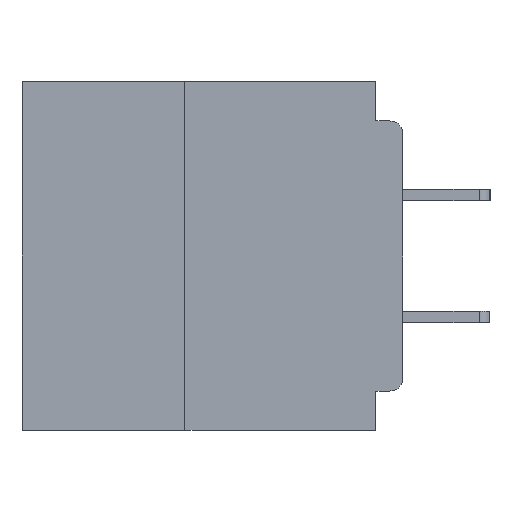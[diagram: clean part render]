
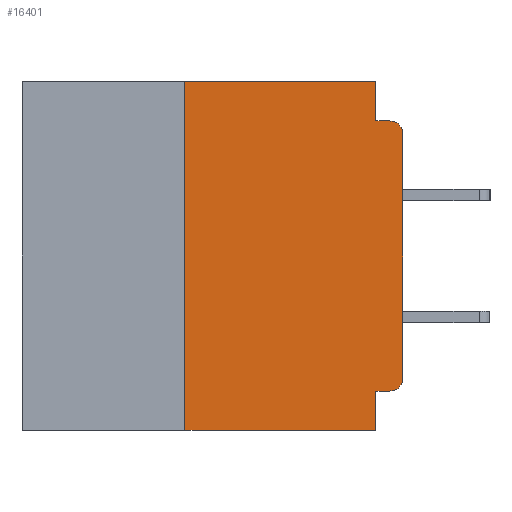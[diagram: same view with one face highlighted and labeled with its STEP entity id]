
A CAD part, left-side view. The second image highlights one B-rep face of the part: STEP entity #16401.
In plain terms, the highlighted planar face has unit normal (-1, 0, 0).
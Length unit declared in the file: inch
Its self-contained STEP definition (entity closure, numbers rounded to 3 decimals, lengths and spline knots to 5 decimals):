
#116 = ORIENTED_EDGE ( 'NONE', *, *, #17835, .T. ) ;
#243 = DIRECTION ( 'NONE',  ( 1., 0., 0. ) ) ;
#404 = ORIENTED_EDGE ( 'NONE', *, *, #12622, .F. ) ;
#516 = DIRECTION ( 'NONE',  ( 0., -1., 0. ) ) ;
#699 = ORIENTED_EDGE ( 'NONE', *, *, #6581, .F. ) ;
#731 = CARTESIAN_POINT ( 'NONE',  ( 0., 0.437, 0. ) ) ;
#815 = CARTESIAN_POINT ( 'NONE',  ( 0., 0.031, -0.355 ) ) ;
#990 = VECTOR ( 'NONE', #34833, 39.37008 ) ;
#2074 = EDGE_CURVE ( 'NONE', #23685, #32540, #9881, .T. ) ;
#2911 = EDGE_CURVE ( 'NONE', #17090, #6119, #20138, .T. ) ;
#3537 = CARTESIAN_POINT ( 'NONE',  ( 0., 0.031, 0. ) ) ;
#3627 = EDGE_CURVE ( 'NONE', #30890, #26163, #35342, .T. ) ;
#3817 = FACE_OUTER_BOUND ( 'NONE', #31645, .T. ) ;
#4033 = CARTESIAN_POINT ( 'NONE',  ( 0., 0.015, -0.355 ) ) ;
#4308 = ORIENTED_EDGE ( 'NONE', *, *, #5670, .F. ) ;
#4828 = ORIENTED_EDGE ( 'NONE', *, *, #32308, .F. ) ;
#4976 = VERTEX_POINT ( 'NONE', #22379 ) ;
#5037 = VECTOR ( 'NONE', #11002, 39.37008 ) ;
#5136 = VECTOR ( 'NONE', #11388, 39.37008 ) ;
#5670 = EDGE_CURVE ( 'NONE', #26163, #34855, #36086, .T. ) ;
#6070 = CARTESIAN_POINT ( 'NONE',  ( 0., 0.437, 0. ) ) ;
#6119 = VERTEX_POINT ( 'NONE', #20509 ) ;
#6156 = DIRECTION ( 'NONE',  ( -1., 0., 0. ) ) ;
#6455 = CARTESIAN_POINT ( 'NONE',  ( 0., 0.437, -0.4 ) ) ;
#6581 = EDGE_CURVE ( 'NONE', #4976, #35070, #22081, .T. ) ;
#9729 = CARTESIAN_POINT ( 'NONE',  ( 0., 0.031, -0.4 ) ) ;
#9881 = LINE ( 'NONE', #731, #30700 ) ;
#9949 = AXIS2_PLACEMENT_3D ( 'NONE', #23336, #6156, #26182 ) ;
#11002 = DIRECTION ( 'NONE',  ( 0., 0., -1. ) ) ;
#11388 = DIRECTION ( 'NONE',  ( 0., 1., 0. ) ) ;
#11932 = CARTESIAN_POINT ( 'NONE',  ( 0., 0., -0.355 ) ) ;
#12227 = ORIENTED_EDGE ( 'NONE', *, *, #3627, .F. ) ;
#12308 = LINE ( 'NONE', #6455, #25605 ) ;
#12622 = EDGE_CURVE ( 'NONE', #32540, #4976, #33221, .T. ) ;
#13429 = CARTESIAN_POINT ( 'NONE',  ( 0., 0.25, -0.4 ) ) ;
#13661 = VECTOR ( 'NONE', #23014, 39.37008 ) ;
#15218 = DIRECTION ( 'NONE',  ( 0., 0., 1. ) ) ;
#15325 = CARTESIAN_POINT ( 'NONE',  ( 0., 0.25, 0. ) ) ;
#15839 = DIRECTION ( 'NONE',  ( -1., 0., 0. ) ) ;
#16401 = ADVANCED_FACE ( 'NONE', ( #3817 ), #28958, .F. ) ;
#16476 = ORIENTED_EDGE ( 'NONE', *, *, #19208, .T. ) ;
#17090 = VERTEX_POINT ( 'NONE', #26309 ) ;
#17835 = EDGE_CURVE ( 'NONE', #6119, #35070, #34373, .T. ) ;
#18929 = ORIENTED_EDGE ( 'NONE', *, *, #35498, .T. ) ;
#19208 = EDGE_CURVE ( 'NONE', #28558, #34855, #12308, .T. ) ;
#19770 = VECTOR ( 'NONE', #15218, 39.37008 ) ;
#20138 = LINE ( 'NONE', #24200, #26715 ) ;
#20509 = CARTESIAN_POINT ( 'NONE',  ( 0., 0., -0.06 ) ) ;
#20597 = DIRECTION ( 'NONE',  ( 0., 0., -1. ) ) ;
#20950 = DIRECTION ( 'NONE',  ( 0., -1., 0. ) ) ;
#21707 = ORIENTED_EDGE ( 'NONE', *, *, #2911, .T. ) ;
#22081 = LINE ( 'NONE', #36866, #13661 ) ;
#22379 = CARTESIAN_POINT ( 'NONE',  ( 0., 0.031, -0.045 ) ) ;
#23014 = DIRECTION ( 'NONE',  ( 0., -1., 0. ) ) ;
#23336 = CARTESIAN_POINT ( 'NONE',  ( 0., 0.015, -0.06 ) ) ;
#23685 = VERTEX_POINT ( 'NONE', #15325 ) ;
#23905 = DIRECTION ( 'NONE',  ( 0., 0., 1. ) ) ;
#24200 = CARTESIAN_POINT ( 'NONE',  ( 0., 0., 0. ) ) ;
#24721 = CIRCLE ( 'NONE', #29258, 0.015 ) ;
#24935 = CARTESIAN_POINT ( 'NONE',  ( 0., 0.031, 0. ) ) ;
#25605 = VECTOR ( 'NONE', #20950, 39.37008 ) ;
#26163 = VERTEX_POINT ( 'NONE', #815 ) ;
#26182 = DIRECTION ( 'NONE',  ( 0., 0., -1. ) ) ;
#26309 = CARTESIAN_POINT ( 'NONE',  ( 0., 0., -0.34 ) ) ;
#26715 = VECTOR ( 'NONE', #23905, 39.37008 ) ;
#26828 = AXIS2_PLACEMENT_3D ( 'NONE', #6070, #243, #20597 ) ;
#27618 = LINE ( 'NONE', #34825, #19770 ) ;
#28558 = VERTEX_POINT ( 'NONE', #13429 ) ;
#28958 = PLANE ( 'NONE',  #26828 ) ;
#29258 = AXIS2_PLACEMENT_3D ( 'NONE', #32672, #15839, #35416 ) ;
#29561 = ORIENTED_EDGE ( 'NONE', *, *, #2074, .F. ) ;
#30700 = VECTOR ( 'NONE', #516, 39.37008 ) ;
#30890 = VERTEX_POINT ( 'NONE', #4033 ) ;
#31645 = EDGE_LOOP ( 'NONE', ( #21707, #116, #699, #404, #29561, #4828, #16476, #4308, #12227, #18929 ) ) ;
#32308 = EDGE_CURVE ( 'NONE', #28558, #23685, #27618, .T. ) ;
#32361 = CARTESIAN_POINT ( 'NONE',  ( 0., 0.031, -0.4 ) ) ;
#32540 = VERTEX_POINT ( 'NONE', #24935 ) ;
#32672 = CARTESIAN_POINT ( 'NONE',  ( 0., 0.015, -0.34 ) ) ;
#33221 = LINE ( 'NONE', #3537, #990 ) ;
#33427 = CARTESIAN_POINT ( 'NONE',  ( 0., 0.015, -0.045 ) ) ;
#34373 = CIRCLE ( 'NONE', #9949, 0.015 ) ;
#34825 = CARTESIAN_POINT ( 'NONE',  ( 0., 0.25, -0.4 ) ) ;
#34833 = DIRECTION ( 'NONE',  ( 0., 0., -1. ) ) ;
#34855 = VERTEX_POINT ( 'NONE', #32361 ) ;
#35070 = VERTEX_POINT ( 'NONE', #33427 ) ;
#35342 = LINE ( 'NONE', #11932, #5136 ) ;
#35416 = DIRECTION ( 'NONE',  ( 0., 0., -1. ) ) ;
#35498 = EDGE_CURVE ( 'NONE', #30890, #17090, #24721, .T. ) ;
#36086 = LINE ( 'NONE', #9729, #5037 ) ;
#36866 = CARTESIAN_POINT ( 'NONE',  ( 0., 0., -0.045 ) ) ;
